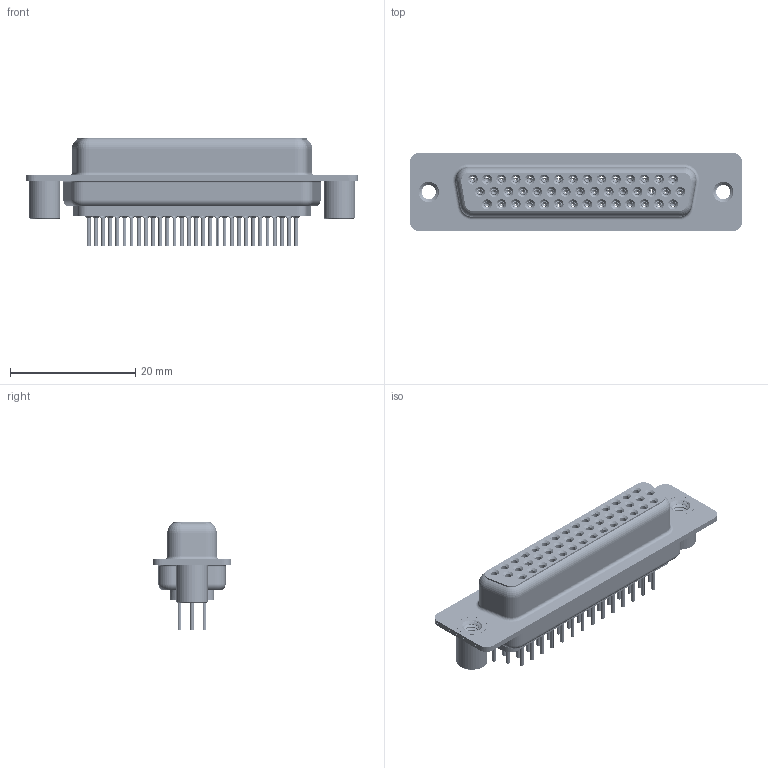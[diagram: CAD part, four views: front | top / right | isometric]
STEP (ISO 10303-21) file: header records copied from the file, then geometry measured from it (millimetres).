
FILE_DESCRIPTION (( 'STEP AP203' ), '1' );
FILE_NAME ('638-044-330-049.STEP', '2020-07-18T22:55:09', ( '' ), ( '' ), 'SwSTEP 2.0', 'SolidWorks 2020', '' );
FILE_SCHEMA (( 'CONFIG_CONTROL_DESIGN' ));
Length unit declared in the file: millimetre
Products named in the file (8): 638-044-330-049; 638 Shell Front_44 Contacts; 638 Contact Row 3_30; 638 Housing_44 Contacts; 638 Shell Rear_44 Contacts; 638 4-40 Threaded Standoff BS; 638 Contact Row 1_30; 638 Contact Row 2_30
Assembly tree (49 placements, depth 2):
  638-044-330-049
    638 Housing_44 Contacts
    638 Shell Front_44 Contacts
    638 Shell Rear_44 Contacts
    638 Contact Row 1_30  x15
    638 Contact Row 2_30  x15
    638 Contact Row 3_30  x14
    638 4-40 Threaded Standoff BS  x2
Bounding box: 53.04 x 12.6 x 17.3 mm (x, y, z)
Volume: 3359.3 mm3; surface area: 12940.3 mm2
Topology: 49 solids, 49 shells, 5889 faces, 15005 edges, 9313 vertices
Faces by surface type: cylinder 1609, plane 1431, torus 1201, bspline 886, cone 762
Entity records: 40440 total; most frequent: CARTESIAN_POINT 11154, DIRECTION 6045, ORIENTED_EDGE 5482, EDGE_CURVE 2741, AXIS2_PLACEMENT_3D 2544, VERTEX_POINT 1731, EDGE_LOOP 1408, CIRCLE 1390
